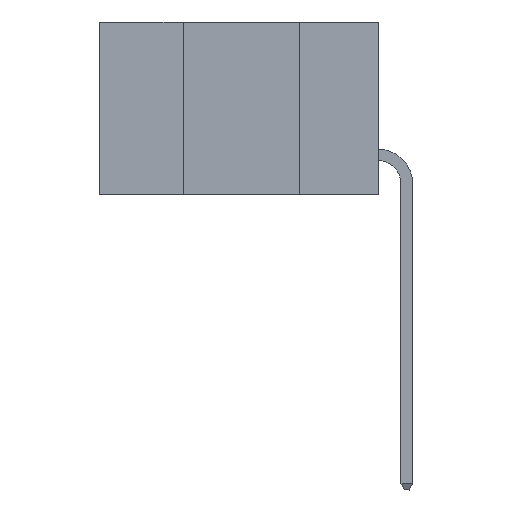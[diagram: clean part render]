
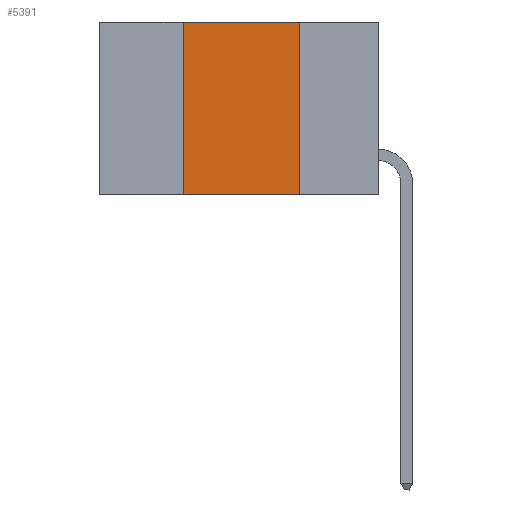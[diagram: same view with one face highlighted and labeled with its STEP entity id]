
A CAD part, left-side view. The second image highlights one B-rep face of the part: STEP entity #5391.
In plain terms, the highlighted planar face has unit normal (-1, 0, 0).
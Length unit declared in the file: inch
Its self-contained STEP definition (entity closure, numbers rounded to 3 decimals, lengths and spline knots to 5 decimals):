
#50 = CARTESIAN_POINT ( 'NONE',  ( 0., 0.17, -0.37 ) ) ;
#224 = LINE ( 'NONE', #3817, #12347 ) ;
#462 = EDGE_CURVE ( 'NONE', #2722, #7756, #224, .T. ) ;
#937 = ORIENTED_EDGE ( 'NONE', *, *, #462, .F. ) ;
#1728 = EDGE_CURVE ( 'NONE', #10508, #7756, #16447, .T. ) ;
#1888 = LINE ( 'NONE', #4336, #18149 ) ;
#2502 = EDGE_CURVE ( 'NONE', #7668, #2722, #1888, .T. ) ;
#2722 = VERTEX_POINT ( 'NONE', #18833 ) ;
#3005 = DIRECTION ( 'NONE',  ( 1., 0., 0. ) ) ;
#3817 = CARTESIAN_POINT ( 'NONE',  ( 0., 0.17, 0. ) ) ;
#3822 = DIRECTION ( 'NONE',  ( 0., 0., -1. ) ) ;
#4191 = DIRECTION ( 'NONE',  ( 0., -1., 0. ) ) ;
#4336 = CARTESIAN_POINT ( 'NONE',  ( 0., 0.6, 0. ) ) ;
#4348 = DIRECTION ( 'NONE',  ( 0., -1., 0. ) ) ;
#5027 = CARTESIAN_POINT ( 'NONE',  ( 0., 0.6, -0.37 ) ) ;
#5391 = ADVANCED_FACE ( 'NONE', ( #9702 ), #9356, .F. ) ;
#5413 = CARTESIAN_POINT ( 'NONE',  ( 0., 0.42, -0.37 ) ) ;
#7668 = VERTEX_POINT ( 'NONE', #20239 ) ;
#7756 = VERTEX_POINT ( 'NONE', #50 ) ;
#8325 = CARTESIAN_POINT ( 'NONE',  ( 0., 0.42, 0. ) ) ;
#9356 = PLANE ( 'NONE',  #11841 ) ;
#9452 = ORIENTED_EDGE ( 'NONE', *, *, #2502, .F. ) ;
#9702 = FACE_OUTER_BOUND ( 'NONE', #18885, .T. ) ;
#10508 = VERTEX_POINT ( 'NONE', #5413 ) ;
#11156 = ORIENTED_EDGE ( 'NONE', *, *, #13366, .F. ) ;
#11464 = DIRECTION ( 'NONE',  ( 0., 0., 1. ) ) ;
#11595 = ORIENTED_EDGE ( 'NONE', *, *, #1728, .T. ) ;
#11841 = AXIS2_PLACEMENT_3D ( 'NONE', #12461, #3005, #14055 ) ;
#12290 = VECTOR ( 'NONE', #4348, 39.37008 ) ;
#12347 = VECTOR ( 'NONE', #3822, 39.37008 ) ;
#12461 = CARTESIAN_POINT ( 'NONE',  ( 0., 0.6, 0. ) ) ;
#13366 = EDGE_CURVE ( 'NONE', #10508, #7668, #15975, .T. ) ;
#14055 = DIRECTION ( 'NONE',  ( 0., 0., -1. ) ) ;
#15975 = LINE ( 'NONE', #8325, #19084 ) ;
#16447 = LINE ( 'NONE', #5027, #12290 ) ;
#18149 = VECTOR ( 'NONE', #4191, 39.37008 ) ;
#18833 = CARTESIAN_POINT ( 'NONE',  ( 0., 0.17, 0. ) ) ;
#18885 = EDGE_LOOP ( 'NONE', ( #937, #9452, #11156, #11595 ) ) ;
#19084 = VECTOR ( 'NONE', #11464, 39.37008 ) ;
#20239 = CARTESIAN_POINT ( 'NONE',  ( 0., 0.42, 0. ) ) ;
